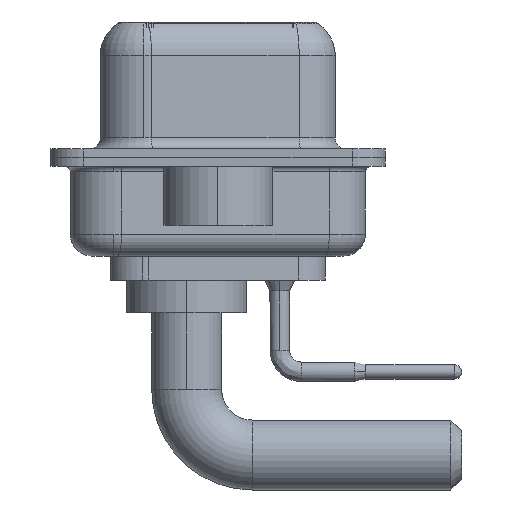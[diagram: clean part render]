
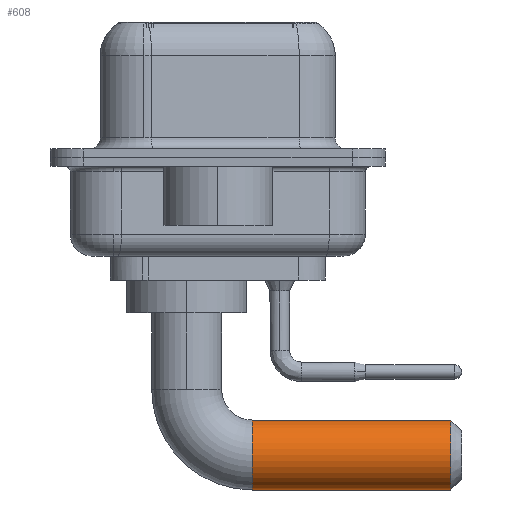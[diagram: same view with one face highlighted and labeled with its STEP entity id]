
A CAD part, left-side view. The second image highlights one B-rep face of the part: STEP entity #608.
In plain terms, the highlighted cylindrical face has radius 1.6 mm (diameter 3.2 mm), a partial arc.
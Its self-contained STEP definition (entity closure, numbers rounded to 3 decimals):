
#608 = ADVANCED_FACE ( 'NONE', ( #14650 ), #14765, .T. ) ;
#1005 = EDGE_CURVE ( 'NONE', #8365, #2802, #6762, .T. ) ;
#1140 = AXIS2_PLACEMENT_3D ( 'NONE', #6336, #8057, #1182 ) ;
#1182 = DIRECTION ( 'NONE',  ( -1., 0., 0. ) ) ;
#1646 = EDGE_CURVE ( 'NONE', #2497, #8365, #6736, .T. ) ;
#2020 = VERTEX_POINT ( 'NONE', #9496 ) ;
#2497 = VERTEX_POINT ( 'NONE', #19484 ) ;
#2802 = VERTEX_POINT ( 'NONE', #20823 ) ;
#2874 = AXIS2_PLACEMENT_3D ( 'NONE', #18207, #4859, #9181 ) ;
#2984 = DIRECTION ( 'NONE',  ( 0., -1., 0. ) ) ;
#2989 = DIRECTION ( 'NONE',  ( 0., 0., -1. ) ) ;
#3236 = ORIENTED_EDGE ( 'NONE', *, *, #11736, .T. ) ;
#4859 = DIRECTION ( 'NONE',  ( 0., -1., 0. ) ) ;
#6336 = CARTESIAN_POINT ( 'NONE',  ( 0., -3., -6.5 ) ) ;
#6439 = ORIENTED_EDGE ( 'NONE', *, *, #1646, .T. ) ;
#6736 = LINE ( 'NONE', #7056, #19149 ) ;
#6762 = CIRCLE ( 'NONE', #16798, 1.6 ) ;
#7056 = CARTESIAN_POINT ( 'NONE',  ( 0., -3., -8.1 ) ) ;
#7945 = CARTESIAN_POINT ( 'NONE',  ( 0., -12.07, -6.5 ) ) ;
#8057 = DIRECTION ( 'NONE',  ( 0., -1., 0. ) ) ;
#8365 = VERTEX_POINT ( 'NONE', #13379 ) ;
#9181 = DIRECTION ( 'NONE',  ( 0., 0., -1. ) ) ;
#9496 = CARTESIAN_POINT ( 'NONE',  ( 0., -3., -4.9 ) ) ;
#9549 = LINE ( 'NONE', #9657, #16664 ) ;
#9657 = CARTESIAN_POINT ( 'NONE',  ( 0., -3., -4.9 ) ) ;
#10435 = CIRCLE ( 'NONE', #1140, 1.6 ) ;
#11409 = DIRECTION ( 'NONE',  ( 0., 1., 0. ) ) ;
#11695 = DIRECTION ( 'NONE',  ( 0., -1., 0. ) ) ;
#11736 = EDGE_CURVE ( 'NONE', #2020, #2497, #10435, .T. ) ;
#12195 = EDGE_LOOP ( 'NONE', ( #15371, #3236, #6439, #14732 ) ) ;
#13379 = CARTESIAN_POINT ( 'NONE',  ( 0., -12.07, -8.1 ) ) ;
#14614 = EDGE_CURVE ( 'NONE', #2020, #2802, #9549, .T. ) ;
#14650 = FACE_OUTER_BOUND ( 'NONE', #12195, .T. ) ;
#14732 = ORIENTED_EDGE ( 'NONE', *, *, #1005, .T. ) ;
#14765 = CYLINDRICAL_SURFACE ( 'NONE', #2874, 1.6 ) ;
#15371 = ORIENTED_EDGE ( 'NONE', *, *, #14614, .F. ) ;
#16664 = VECTOR ( 'NONE', #2984, 1000. ) ;
#16798 = AXIS2_PLACEMENT_3D ( 'NONE', #7945, #11409, #2989 ) ;
#18207 = CARTESIAN_POINT ( 'NONE',  ( 0., -3., -6.5 ) ) ;
#19149 = VECTOR ( 'NONE', #11695, 1000. ) ;
#19484 = CARTESIAN_POINT ( 'NONE',  ( 0., -3., -8.1 ) ) ;
#20823 = CARTESIAN_POINT ( 'NONE',  ( 0., -12.07, -4.9 ) ) ;
